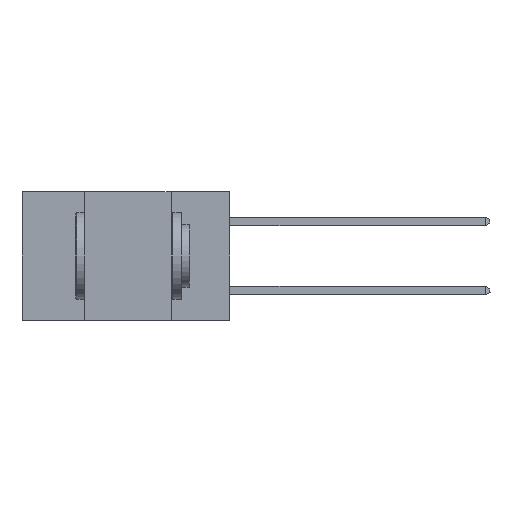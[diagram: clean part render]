
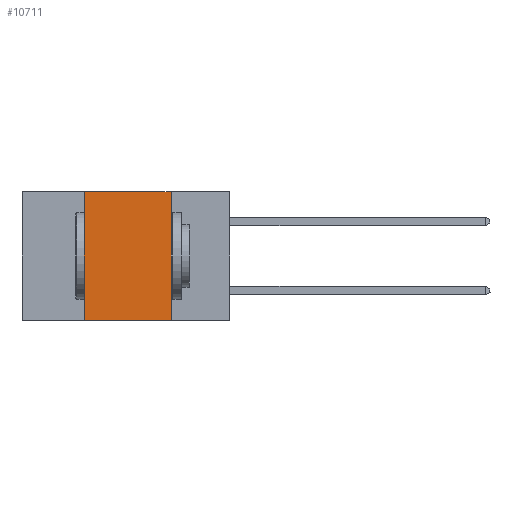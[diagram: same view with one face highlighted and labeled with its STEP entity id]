
A CAD part, left-side view. The second image highlights one B-rep face of the part: STEP entity #10711.
In plain terms, the highlighted planar face has unit normal (-1, 0, 0).
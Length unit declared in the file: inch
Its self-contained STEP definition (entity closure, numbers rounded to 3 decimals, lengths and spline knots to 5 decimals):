
#352 = EDGE_CURVE ( 'NONE', #15048, #25678, #6050, .T. ) ;
#3415 = CARTESIAN_POINT ( 'NONE',  ( 0., 0.42, 0. ) ) ;
#5214 = CARTESIAN_POINT ( 'NONE',  ( 0., 0.6, 0. ) ) ;
#5730 = VECTOR ( 'NONE', #16975, 39.37008 ) ;
#5886 = VECTOR ( 'NONE', #15925, 39.37008 ) ;
#6050 = LINE ( 'NONE', #12556, #15253 ) ;
#8039 = CARTESIAN_POINT ( 'NONE',  ( 0., 0.17, 0. ) ) ;
#9770 = DIRECTION ( 'NONE',  ( 1., 0., 0. ) ) ;
#10711 = ADVANCED_FACE ( 'NONE', ( #26302 ), #16405, .F. ) ;
#11016 = VECTOR ( 'NONE', #24738, 39.37008 ) ;
#11367 = LINE ( 'NONE', #29092, #11016 ) ;
#12040 = DIRECTION ( 'NONE',  ( 0., 0., -1. ) ) ;
#12556 = CARTESIAN_POINT ( 'NONE',  ( 0., 0.6, 0. ) ) ;
#14020 = CARTESIAN_POINT ( 'NONE',  ( 0., 0.17, -0.37 ) ) ;
#14575 = LINE ( 'NONE', #8039, #5730 ) ;
#14926 = EDGE_CURVE ( 'NONE', #19388, #18533, #15807, .T. ) ;
#15013 = DIRECTION ( 'NONE',  ( 0., -1., 0. ) ) ;
#15048 = VERTEX_POINT ( 'NONE', #3415 ) ;
#15253 = VECTOR ( 'NONE', #15013, 39.37008 ) ;
#15614 = CARTESIAN_POINT ( 'NONE',  ( 0., 0.42, -0.37 ) ) ;
#15807 = LINE ( 'NONE', #26957, #5886 ) ;
#15925 = DIRECTION ( 'NONE',  ( 0., -1., 0. ) ) ;
#16245 = AXIS2_PLACEMENT_3D ( 'NONE', #5214, #9770, #12040 ) ;
#16288 = ORIENTED_EDGE ( 'NONE', *, *, #14926, .T. ) ;
#16405 = PLANE ( 'NONE',  #16245 ) ;
#16975 = DIRECTION ( 'NONE',  ( 0., 0., -1. ) ) ;
#17678 = ORIENTED_EDGE ( 'NONE', *, *, #352, .F. ) ;
#18533 = VERTEX_POINT ( 'NONE', #14020 ) ;
#18589 = EDGE_CURVE ( 'NONE', #25678, #18533, #14575, .T. ) ;
#19388 = VERTEX_POINT ( 'NONE', #15614 ) ;
#20191 = ORIENTED_EDGE ( 'NONE', *, *, #18589, .F. ) ;
#22018 = ORIENTED_EDGE ( 'NONE', *, *, #22092, .F. ) ;
#22092 = EDGE_CURVE ( 'NONE', #19388, #15048, #11367, .T. ) ;
#22905 = CARTESIAN_POINT ( 'NONE',  ( 0., 0.17, 0. ) ) ;
#24738 = DIRECTION ( 'NONE',  ( 0., 0., 1. ) ) ;
#25678 = VERTEX_POINT ( 'NONE', #22905 ) ;
#26110 = EDGE_LOOP ( 'NONE', ( #20191, #17678, #22018, #16288 ) ) ;
#26302 = FACE_OUTER_BOUND ( 'NONE', #26110, .T. ) ;
#26957 = CARTESIAN_POINT ( 'NONE',  ( 0., 0.6, -0.37 ) ) ;
#29092 = CARTESIAN_POINT ( 'NONE',  ( 0., 0.42, 0. ) ) ;
